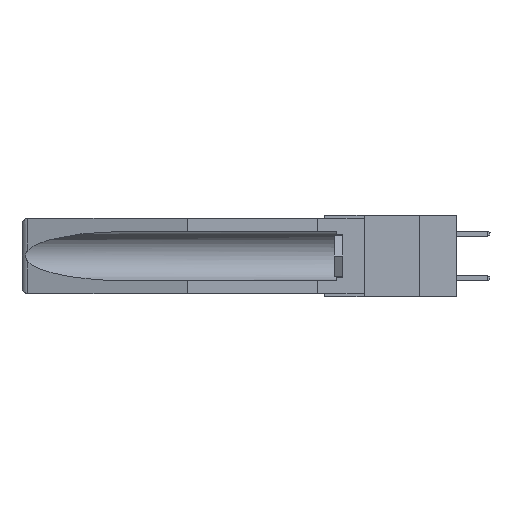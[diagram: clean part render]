
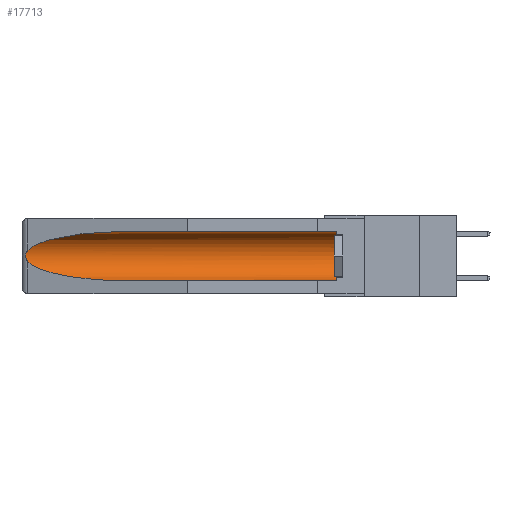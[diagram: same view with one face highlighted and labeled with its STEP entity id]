
A CAD part, left-side view. The second image highlights one B-rep face of the part: STEP entity #17713.
In plain terms, the highlighted cylindrical face has radius 2.857 mm (diameter 5.715 mm), a partial arc.
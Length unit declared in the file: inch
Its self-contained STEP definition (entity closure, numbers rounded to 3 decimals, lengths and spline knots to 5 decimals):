
#161 = EDGE_CURVE ( 'NONE', #20412, #7022, #22811, .T. ) ;
#196 = EDGE_CURVE ( 'NONE', #8904, #20412, #15106, .T. ) ;
#389 = EDGE_CURVE ( 'NONE', #17973, #13082, #11373, .T. ) ;
#553 = ORIENTED_EDGE ( 'NONE', *, *, #2606, .F. ) ;
#586 = DIRECTION ( 'NONE',  ( 0., 0., 1. ) ) ;
#2056 = CARTESIAN_POINT ( 'NONE',  ( 0.155, 1.07973, -0.059 ) ) ;
#2211 = CARTESIAN_POINT ( 'NONE',  ( 0.26537, 1.52718, -0.19328 ) ) ;
#2339 = ORIENTED_EDGE ( 'NONE', *, *, #389, .T. ) ;
#2504 = CARTESIAN_POINT ( 'NONE',  ( 0.155, 0.126, -0.1715 ) ) ;
#2532 = CARTESIAN_POINT ( 'NONE',  ( 0.2673, 1.5327, -0.16383 ) ) ;
#2606 = EDGE_CURVE ( 'NONE', #14055, #7022, #4300, .T. ) ;
#2812 = ORIENTED_EDGE ( 'NONE', *, *, #17779, .T. ) ;
#3460 = CARTESIAN_POINT ( 'NONE',  ( 0.155, 1.07973, -0.059 ) ) ;
#3799 = EDGE_CURVE ( 'NONE', #13082, #8904, #19510, .T. ) ;
#4287 = CARTESIAN_POINT ( 'NONE',  ( 0.155, 1.07973, -0.284 ) ) ;
#4300 = LINE ( 'NONE', #18066, #22061 ) ;
#4634 = CARTESIAN_POINT ( 'NONE',  ( 0.155, 1.07973, -0.284 ) ) ;
#5410 = ORIENTED_EDGE ( 'NONE', *, *, #196, .T. ) ;
#5609 = CARTESIAN_POINT ( 'NONE',  ( 0.21114, 1.30732, -0.059 ) ) ;
#5941 = CARTESIAN_POINT ( 'NONE',  ( 0.2675, 1.53308, -0.16763 ) ) ;
#6092 = CARTESIAN_POINT ( 'NONE',  ( 0.2675, 1.53308, -0.17534 ) ) ;
#7022 = VERTEX_POINT ( 'NONE', #4634 ) ;
#7051 = DIRECTION ( 'NONE',  ( 0., 0., 1. ) ) ;
#7237 = CARTESIAN_POINT ( 'NONE',  ( 0.26537, 1.52718, -0.14972 ) ) ;
#7556 = FACE_OUTER_BOUND ( 'NONE', #19495, .T. ) ;
#7563 = AXIS2_PLACEMENT_3D ( 'NONE', #15801, #10543, #7051 ) ;
#7711 = CARTESIAN_POINT ( 'NONE',  ( 0.2673, 1.53269, -0.17917 ) ) ;
#7773 = CARTESIAN_POINT ( 'NONE',  ( 0.155, 0.126, -0.284 ) ) ;
#7945 = CARTESIAN_POINT ( 'NONE',  ( 0.26655, 1.53094, -0.18657 ) ) ;
#8020 = CARTESIAN_POINT ( 'NONE',  ( 0.26537, 1.52718, -0.19328 ) ) ;
#8769 = AXIS2_PLACEMENT_3D ( 'NONE', #2504, #21793, #586 ) ;
#8904 = VERTEX_POINT ( 'NONE', #7237 ) ;
#9020 = DIRECTION ( 'NONE',  ( 0., 1., 0. ) ) ;
#10441 = ORIENTED_EDGE ( 'NONE', *, *, #161, .T. ) ;
#10543 = DIRECTION ( 'NONE',  ( 0., 1., 0. ) ) ;
#10891 = ORIENTED_EDGE ( 'NONE', *, *, #3799, .T. ) ;
#11178 = CARTESIAN_POINT ( 'NONE',  ( 0.26597, 1.52961, -0.15275 ) ) ;
#11373 = LINE ( 'NONE', #14207, #22681 ) ;
#11485 = CARTESIAN_POINT ( 'NONE',  ( 0.26537, 1.52718, -0.19328 ) ) ;
#12964 = CARTESIAN_POINT ( 'NONE',  ( 0.21114, 1.30732, -0.284 ) ) ;
#13082 = VERTEX_POINT ( 'NONE', #3460 ) ;
#13117 = CARTESIAN_POINT ( 'NONE',  ( 0.26537, 1.52718, -0.14972 ) ) ;
#14055 = VERTEX_POINT ( 'NONE', #7773 ) ;
#14207 = CARTESIAN_POINT ( 'NONE',  ( 0.155, -0.30754, -0.059 ) ) ;
#14744 = CARTESIAN_POINT ( 'NONE',  ( 0.26654, 1.53092, -0.15636 ) ) ;
#15106 = B_SPLINE_CURVE_WITH_KNOTS ( 'NONE', 3,
 ( #13117, #11178, #14744, #2532, #5941, #6092, #7711, #7945, #22119, #11485 ),
 .UNSPECIFIED., .F., .F.,
 ( 4, 2, 2, 2, 4 ),
 ( 0., 0.00029, 0.00058, 0.00087, 0.00117 ),
 .UNSPECIFIED. ) ;
#15590 = CIRCLE ( 'NONE', #8769, 0.1125 ) ;
#15801 = CARTESIAN_POINT ( 'NONE',  ( 0.155, -0.30754, -0.1715 ) ) ;
#17713 = ADVANCED_FACE ( 'NONE', ( #7556 ), #21137, .F. ) ;
#17779 = EDGE_CURVE ( 'NONE', #14055, #17973, #15590, .T. ) ;
#17966 = CARTESIAN_POINT ( 'NONE',  ( 0.25451, 1.48313, -0.09465 ) ) ;
#17973 = VERTEX_POINT ( 'NONE', #20592 ) ;
#18066 = CARTESIAN_POINT ( 'NONE',  ( 0.155, -0.30754, -0.284 ) ) ;
#18596 = DIRECTION ( 'NONE',  ( 0., 1., 0. ) ) ;
#19495 = EDGE_LOOP ( 'NONE', ( #10891, #5410, #10441, #553, #2812, #2339 ) ) ;
#19510 =( BOUNDED_CURVE ( )  B_SPLINE_CURVE ( 3, ( #2056, #5609, #17966, #21799 ),
 .UNSPECIFIED., .F., .T. ) 
 B_SPLINE_CURVE_WITH_KNOTS ( ( 4, 4 ),
 ( 4.71239, 6.08839 ),
 .UNSPECIFIED. ) 
 CURVE ( )  GEOMETRIC_REPRESENTATION_ITEM ( )  RATIONAL_B_SPLINE_CURVE ( ( 1., 0.848, 0.848, 1. ) ) 
 REPRESENTATION_ITEM ( '' )  );
#20187 = CARTESIAN_POINT ( 'NONE',  ( 0.25451, 1.48313, -0.24835 ) ) ;
#20412 = VERTEX_POINT ( 'NONE', #2211 ) ;
#20592 = CARTESIAN_POINT ( 'NONE',  ( 0.155, 0.126, -0.059 ) ) ;
#21137 = CYLINDRICAL_SURFACE ( 'NONE', #7563, 0.1125 ) ;
#21793 = DIRECTION ( 'NONE',  ( 0., -1., 0. ) ) ;
#21799 = CARTESIAN_POINT ( 'NONE',  ( 0.26537, 1.52718, -0.14972 ) ) ;
#22061 = VECTOR ( 'NONE', #18596, 39.37008 ) ;
#22119 = CARTESIAN_POINT ( 'NONE',  ( 0.26597, 1.5296, -0.19026 ) ) ;
#22681 = VECTOR ( 'NONE', #9020, 39.37008 ) ;
#22811 =( BOUNDED_CURVE ( )  B_SPLINE_CURVE ( 3, ( #8020, #20187, #12964, #4287 ),
 .UNSPECIFIED., .F., .F. ) 
 B_SPLINE_CURVE_WITH_KNOTS ( ( 4, 4 ),
 ( 0.1948, 1.5708 ),
 .UNSPECIFIED. ) 
 CURVE ( )  GEOMETRIC_REPRESENTATION_ITEM ( )  RATIONAL_B_SPLINE_CURVE ( ( 1., 0.848, 0.848, 1. ) ) 
 REPRESENTATION_ITEM ( '' )  );
